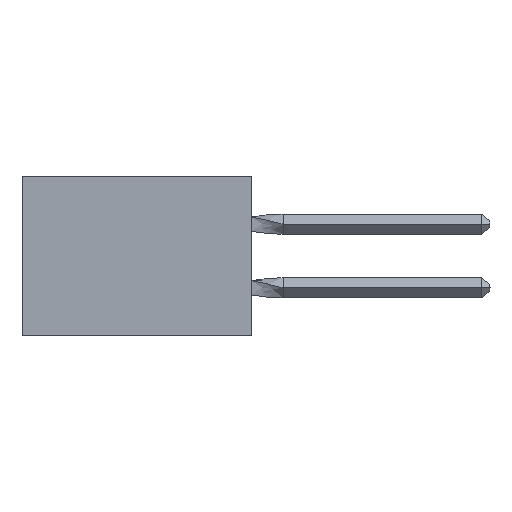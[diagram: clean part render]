
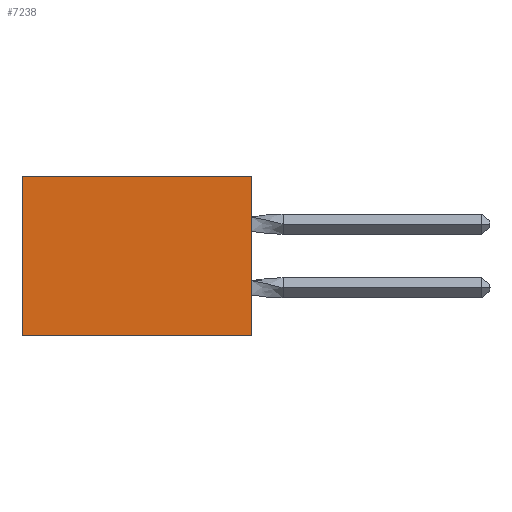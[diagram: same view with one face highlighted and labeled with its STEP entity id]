
A CAD part, left-side view. The second image highlights one B-rep face of the part: STEP entity #7238.
In plain terms, the highlighted planar face has unit normal (-1, 0, 0).
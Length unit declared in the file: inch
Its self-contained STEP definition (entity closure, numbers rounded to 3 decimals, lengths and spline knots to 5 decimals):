
#99 = DIRECTION ( 'NONE',  ( 0., 1., 0. ) ) ;
#483 = DIRECTION ( 'NONE',  ( 0., 0., -1. ) ) ;
#512 = CARTESIAN_POINT ( 'NONE',  ( 0.305, 0., 0. ) ) ;
#604 = VECTOR ( 'NONE', #1996, 39.37008 ) ;
#694 = EDGE_CURVE ( 'NONE', #8500, #6121, #9667, .T. ) ;
#1085 = ORIENTED_EDGE ( 'NONE', *, *, #7451, .T. ) ;
#1601 = DIRECTION ( 'NONE',  ( 1., 0., 0. ) ) ;
#1721 = CARTESIAN_POINT ( 'NONE',  ( 0.305, 0.72, 0. ) ) ;
#1996 = DIRECTION ( 'NONE',  ( 0., 0., -1. ) ) ;
#2082 = LINE ( 'NONE', #6634, #9926 ) ;
#2092 = VERTEX_POINT ( 'NONE', #9712 ) ;
#2920 = CARTESIAN_POINT ( 'NONE',  ( 0.305, 0.72, -0.5 ) ) ;
#3983 = ORIENTED_EDGE ( 'NONE', *, *, #12761, .F. ) ;
#4005 = EDGE_LOOP ( 'NONE', ( #1085, #8112, #3983, #11643 ) ) ;
#5405 = DIRECTION ( 'NONE',  ( 0., 1., 0. ) ) ;
#5785 = LINE ( 'NONE', #2920, #604 ) ;
#5874 = DIRECTION ( 'NONE',  ( 0., 0., -1. ) ) ;
#6121 = VERTEX_POINT ( 'NONE', #1721 ) ;
#6579 = LINE ( 'NONE', #10586, #8836 ) ;
#6634 = CARTESIAN_POINT ( 'NONE',  ( 0.305, 0., -0.5 ) ) ;
#6771 = CARTESIAN_POINT ( 'NONE',  ( 0.305, 0., -0.5 ) ) ;
#7238 = ADVANCED_FACE ( 'NONE', ( #12657 ), #10818, .F. ) ;
#7451 = EDGE_CURVE ( 'NONE', #6121, #2092, #5785, .T. ) ;
#8112 = ORIENTED_EDGE ( 'NONE', *, *, #12621, .F. ) ;
#8500 = VERTEX_POINT ( 'NONE', #512 ) ;
#8836 = VECTOR ( 'NONE', #5405, 39.37008 ) ;
#9667 = LINE ( 'NONE', #11430, #9977 ) ;
#9712 = CARTESIAN_POINT ( 'NONE',  ( 0.305, 0.72, -0.5 ) ) ;
#9926 = VECTOR ( 'NONE', #483, 39.37008 ) ;
#9977 = VECTOR ( 'NONE', #99, 39.37008 ) ;
#10586 = CARTESIAN_POINT ( 'NONE',  ( 0.305, 0., -0.5 ) ) ;
#10653 = VERTEX_POINT ( 'NONE', #12982 ) ;
#10818 = PLANE ( 'NONE',  #12392 ) ;
#11430 = CARTESIAN_POINT ( 'NONE',  ( 0.305, 0., 0. ) ) ;
#11643 = ORIENTED_EDGE ( 'NONE', *, *, #694, .T. ) ;
#12392 = AXIS2_PLACEMENT_3D ( 'NONE', #6771, #1601, #5874 ) ;
#12621 = EDGE_CURVE ( 'NONE', #10653, #2092, #6579, .T. ) ;
#12657 = FACE_OUTER_BOUND ( 'NONE', #4005, .T. ) ;
#12761 = EDGE_CURVE ( 'NONE', #8500, #10653, #2082, .T. ) ;
#12982 = CARTESIAN_POINT ( 'NONE',  ( 0.305, 0., -0.5 ) ) ;
